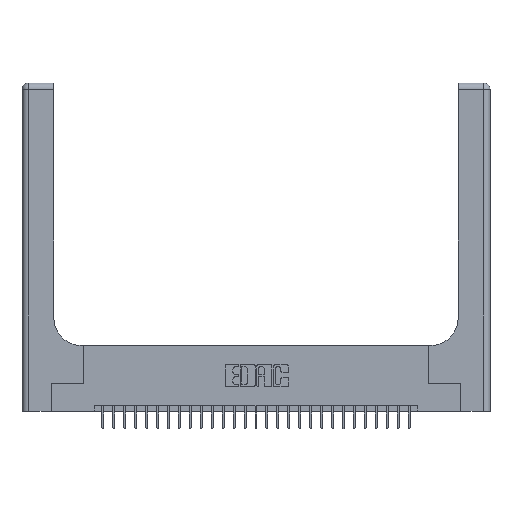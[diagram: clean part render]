
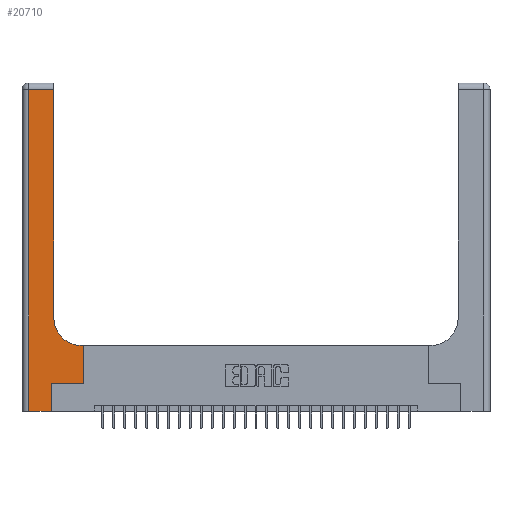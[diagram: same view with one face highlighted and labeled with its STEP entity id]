
A CAD part, top view. The second image highlights one B-rep face of the part: STEP entity #20710.
In plain terms, the highlighted planar face has unit normal (0, 0, 1).
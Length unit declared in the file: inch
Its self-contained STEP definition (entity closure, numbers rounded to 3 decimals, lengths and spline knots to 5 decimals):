
#239 = VERTEX_POINT ( 'NONE', #18167 ) ;
#321 = VERTEX_POINT ( 'NONE', #9781 ) ;
#1504 = EDGE_CURVE ( 'NONE', #18869, #19768, #18211, .T. ) ;
#2193 = DIRECTION ( 'NONE',  ( 1., 0., 0. ) ) ;
#2391 = VECTOR ( 'NONE', #4374, 39.37008 ) ;
#3962 = PLANE ( 'NONE',  #28492 ) ;
#4137 = ORIENTED_EDGE ( 'NONE', *, *, #21694, .T. ) ;
#4312 = DIRECTION ( 'NONE',  ( 0., 1., 0. ) ) ;
#4374 = DIRECTION ( 'NONE',  ( 0., 1., 0. ) ) ;
#4454 = ORIENTED_EDGE ( 'NONE', *, *, #16407, .T. ) ;
#5584 = LINE ( 'NONE', #13817, #2391 ) ;
#5807 = CARTESIAN_POINT ( 'NONE',  ( 0.269, 0., 0.37 ) ) ;
#5935 = DIRECTION ( 'NONE',  ( 0., 0., -1. ) ) ;
#6332 = CARTESIAN_POINT ( 'NONE',  ( 0., 2.94, 0.37 ) ) ;
#6721 = CARTESIAN_POINT ( 'NONE',  ( 0.2915, 2.94, 0.37 ) ) ;
#6977 = VERTEX_POINT ( 'NONE', #6721 ) ;
#7514 = EDGE_CURVE ( 'NONE', #19768, #9394, #29400, .T. ) ;
#8240 = CARTESIAN_POINT ( 'NONE',  ( 0.06, 3., 0.37 ) ) ;
#8533 = DIRECTION ( 'NONE',  ( -1., 0., 0. ) ) ;
#8619 = VERTEX_POINT ( 'NONE', #14248 ) ;
#8916 = EDGE_CURVE ( 'NONE', #24838, #18869, #19278, .T. ) ;
#9376 = AXIS2_PLACEMENT_3D ( 'NONE', #15792, #27432, #2193 ) ;
#9394 = VERTEX_POINT ( 'NONE', #12144 ) ;
#9781 = CARTESIAN_POINT ( 'NONE',  ( 0.269, 0., 0.37 ) ) ;
#10091 = ORIENTED_EDGE ( 'NONE', *, *, #10110, .T. ) ;
#10110 = EDGE_CURVE ( 'NONE', #321, #24838, #29261, .T. ) ;
#10259 = DIRECTION ( 'NONE',  ( 0., 1., 0. ) ) ;
#10364 = VECTOR ( 'NONE', #10576, 39.37008 ) ;
#10576 = DIRECTION ( 'NONE',  ( 0., -1., 0. ) ) ;
#10741 = ORIENTED_EDGE ( 'NONE', *, *, #7514, .T. ) ;
#12144 = CARTESIAN_POINT ( 'NONE',  ( 0.5415, 0.6, 0.37 ) ) ;
#12461 = VECTOR ( 'NONE', #8533, 39.37008 ) ;
#12542 = EDGE_CURVE ( 'NONE', #12735, #239, #17970, .T. ) ;
#12714 = LINE ( 'NONE', #18836, #28554 ) ;
#12735 = VERTEX_POINT ( 'NONE', #16323 ) ;
#13140 = VECTOR ( 'NONE', #13512, 39.37008 ) ;
#13512 = DIRECTION ( 'NONE',  ( 1., 0., 0. ) ) ;
#13817 = CARTESIAN_POINT ( 'NONE',  ( 0.2915, 3., 0.37 ) ) ;
#14248 = CARTESIAN_POINT ( 'NONE',  ( 0.2915, 0.85, 0.37 ) ) ;
#14262 = VECTOR ( 'NONE', #29028, 39.37008 ) ;
#15246 = ORIENTED_EDGE ( 'NONE', *, *, #12542, .T. ) ;
#15792 = CARTESIAN_POINT ( 'NONE',  ( 0.5415, 0.85, 0.37 ) ) ;
#16323 = CARTESIAN_POINT ( 'NONE',  ( 0.06, 2.94, 0.37 ) ) ;
#16407 = EDGE_CURVE ( 'NONE', #6977, #12735, #29044, .T. ) ;
#17852 = CARTESIAN_POINT ( 'NONE',  ( 0.5585, 0.25, 0.37 ) ) ;
#17970 = LINE ( 'NONE', #8240, #10364 ) ;
#18167 = CARTESIAN_POINT ( 'NONE',  ( 0.06, 0., 0.37 ) ) ;
#18211 = LINE ( 'NONE', #29534, #25786 ) ;
#18470 = EDGE_CURVE ( 'NONE', #9394, #8619, #28527, .T. ) ;
#18836 = CARTESIAN_POINT ( 'NONE',  ( 0., 0., 0.37 ) ) ;
#18869 = VERTEX_POINT ( 'NONE', #17852 ) ;
#19278 = LINE ( 'NONE', #29298, #13140 ) ;
#19768 = VERTEX_POINT ( 'NONE', #23450 ) ;
#19812 = CARTESIAN_POINT ( 'NONE',  ( 0.2915, 0.6, 0.37 ) ) ;
#20710 = ADVANCED_FACE ( 'NONE', ( #24351 ), #3962, .F. ) ;
#21694 = EDGE_CURVE ( 'NONE', #239, #321, #12714, .T. ) ;
#22068 = EDGE_LOOP ( 'NONE', ( #27035, #4454, #15246, #4137, #10091, #24778, #28854, #10741, #25417 ) ) ;
#23174 = VECTOR ( 'NONE', #10259, 39.37008 ) ;
#23450 = CARTESIAN_POINT ( 'NONE',  ( 0.5585, 0.6, 0.37 ) ) ;
#23923 = CARTESIAN_POINT ( 'NONE',  ( 0.269, 0.25, 0.37 ) ) ;
#24351 = FACE_OUTER_BOUND ( 'NONE', #22068, .T. ) ;
#24419 = DIRECTION ( 'NONE',  ( -1., 0., 0. ) ) ;
#24778 = ORIENTED_EDGE ( 'NONE', *, *, #8916, .T. ) ;
#24838 = VERTEX_POINT ( 'NONE', #23923 ) ;
#25417 = ORIENTED_EDGE ( 'NONE', *, *, #18470, .T. ) ;
#25786 = VECTOR ( 'NONE', #4312, 39.37008 ) ;
#26591 = CARTESIAN_POINT ( 'NONE',  ( 0., 3., 0.37 ) ) ;
#27035 = ORIENTED_EDGE ( 'NONE', *, *, #28171, .T. ) ;
#27432 = DIRECTION ( 'NONE',  ( 0., 0., -1. ) ) ;
#28141 = DIRECTION ( 'NONE',  ( 1., 0., 0. ) ) ;
#28171 = EDGE_CURVE ( 'NONE', #8619, #6977, #5584, .T. ) ;
#28492 = AXIS2_PLACEMENT_3D ( 'NONE', #26591, #5935, #24419 ) ;
#28527 = CIRCLE ( 'NONE', #9376, 0.25 ) ;
#28554 = VECTOR ( 'NONE', #28141, 39.37008 ) ;
#28854 = ORIENTED_EDGE ( 'NONE', *, *, #1504, .T. ) ;
#29028 = DIRECTION ( 'NONE',  ( -1., 0., 0. ) ) ;
#29044 = LINE ( 'NONE', #6332, #12461 ) ;
#29261 = LINE ( 'NONE', #5807, #23174 ) ;
#29298 = CARTESIAN_POINT ( 'NONE',  ( 0.269, 0.25, 0.37 ) ) ;
#29400 = LINE ( 'NONE', #19812, #14262 ) ;
#29534 = CARTESIAN_POINT ( 'NONE',  ( 0.5585, 0.25, 0.37 ) ) ;
